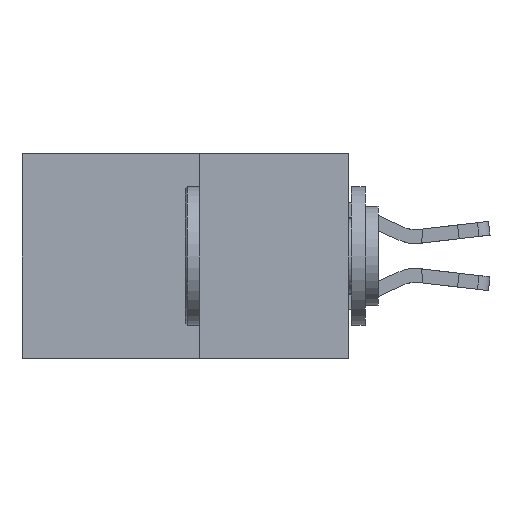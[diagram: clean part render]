
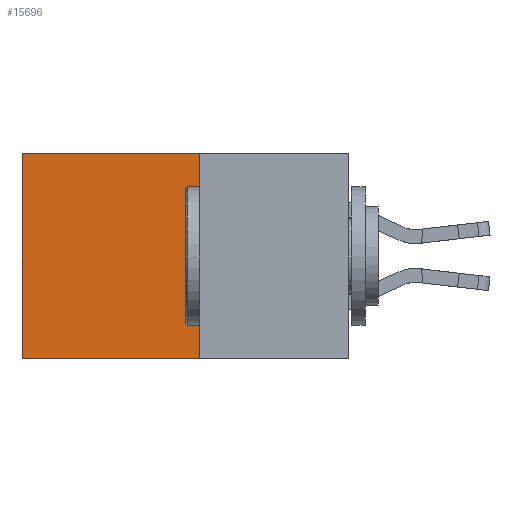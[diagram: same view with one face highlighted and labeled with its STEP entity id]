
A CAD part, left-side view. The second image highlights one B-rep face of the part: STEP entity #15696.
In plain terms, the highlighted planar face has unit normal (-1, 0, 0).
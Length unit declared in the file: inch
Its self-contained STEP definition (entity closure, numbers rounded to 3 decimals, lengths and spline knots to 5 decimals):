
#279 = LINE ( 'NONE', #16870, #16618 ) ;
#673 = ORIENTED_EDGE ( 'NONE', *, *, #6783, .F. ) ;
#675 = EDGE_CURVE ( 'NONE', #792, #1586, #279, .T. ) ;
#792 = VERTEX_POINT ( 'NONE', #7549 ) ;
#886 = VECTOR ( 'NONE', #10662, 39.37008 ) ;
#1248 = EDGE_CURVE ( 'NONE', #12460, #792, #11582, .T. ) ;
#1586 = VERTEX_POINT ( 'NONE', #16259 ) ;
#2524 = DIRECTION ( 'NONE',  ( 1., 0., 0. ) ) ;
#4686 = ORIENTED_EDGE ( 'NONE', *, *, #1248, .T. ) ;
#5192 = PLANE ( 'NONE',  #8605 ) ;
#5245 = CARTESIAN_POINT ( 'NONE',  ( 0.277, 0.27, -0.37 ) ) ;
#5306 = CARTESIAN_POINT ( 'NONE',  ( 0.277, 0.27, 0. ) ) ;
#5529 = DIRECTION ( 'NONE',  ( 0., 1., 0. ) ) ;
#6263 = EDGE_CURVE ( 'NONE', #7207, #1586, #7542, .T. ) ;
#6783 = EDGE_CURVE ( 'NONE', #12460, #7207, #7299, .T. ) ;
#6893 = VECTOR ( 'NONE', #8007, 39.37008 ) ;
#7207 = VERTEX_POINT ( 'NONE', #8413 ) ;
#7299 = LINE ( 'NONE', #7984, #6893 ) ;
#7542 = LINE ( 'NONE', #5245, #14466 ) ;
#7549 = CARTESIAN_POINT ( 'NONE',  ( 0.277, 0.59, 0. ) ) ;
#7984 = CARTESIAN_POINT ( 'NONE',  ( 0.277, 0.27, -0.37 ) ) ;
#8007 = DIRECTION ( 'NONE',  ( 0., 0., -1. ) ) ;
#8413 = CARTESIAN_POINT ( 'NONE',  ( 0.277, 0.27, -0.37 ) ) ;
#8605 = AXIS2_PLACEMENT_3D ( 'NONE', #10536, #2524, #11896 ) ;
#9280 = ORIENTED_EDGE ( 'NONE', *, *, #675, .T. ) ;
#9281 = FACE_OUTER_BOUND ( 'NONE', #15287, .T. ) ;
#10141 = DIRECTION ( 'NONE',  ( 0., 0., -1. ) ) ;
#10536 = CARTESIAN_POINT ( 'NONE',  ( 0.277, 0.27, -0.37 ) ) ;
#10662 = DIRECTION ( 'NONE',  ( 0., 1., 0. ) ) ;
#11582 = LINE ( 'NONE', #5306, #886 ) ;
#11896 = DIRECTION ( 'NONE',  ( 0., 0., -1. ) ) ;
#12460 = VERTEX_POINT ( 'NONE', #14005 ) ;
#13792 = ORIENTED_EDGE ( 'NONE', *, *, #6263, .F. ) ;
#14005 = CARTESIAN_POINT ( 'NONE',  ( 0.277, 0.27, 0. ) ) ;
#14466 = VECTOR ( 'NONE', #5529, 39.37008 ) ;
#15287 = EDGE_LOOP ( 'NONE', ( #9280, #13792, #673, #4686 ) ) ;
#15696 = ADVANCED_FACE ( 'NONE', ( #9281 ), #5192, .F. ) ;
#16259 = CARTESIAN_POINT ( 'NONE',  ( 0.277, 0.59, -0.37 ) ) ;
#16618 = VECTOR ( 'NONE', #10141, 39.37008 ) ;
#16870 = CARTESIAN_POINT ( 'NONE',  ( 0.277, 0.59, -0.37 ) ) ;
